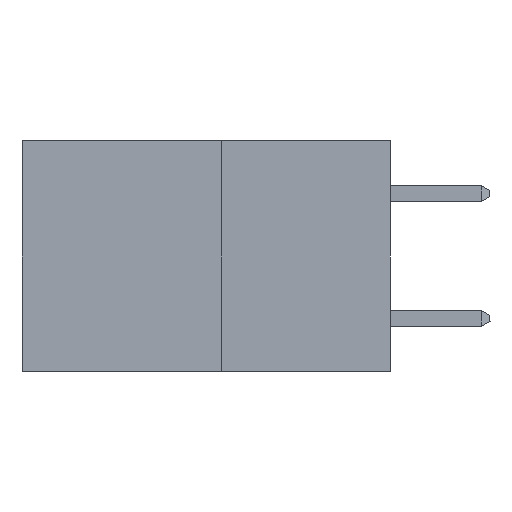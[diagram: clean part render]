
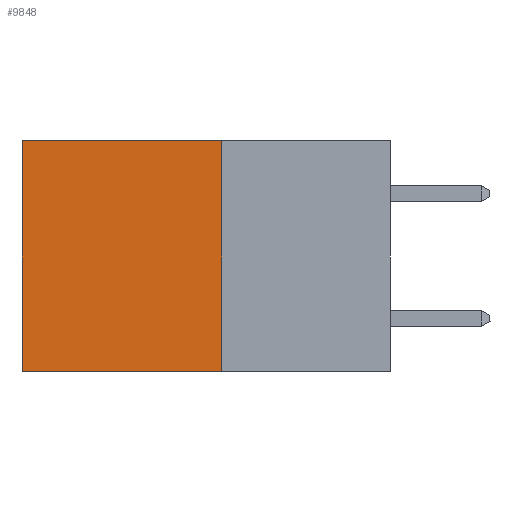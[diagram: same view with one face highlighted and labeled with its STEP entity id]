
A CAD part, left-side view. The second image highlights one B-rep face of the part: STEP entity #9848.
In plain terms, the highlighted planar face has unit normal (-1, 0, 0).
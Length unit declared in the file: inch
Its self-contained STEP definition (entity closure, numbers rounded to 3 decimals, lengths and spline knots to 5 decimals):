
#605 = ORIENTED_EDGE ( 'NONE', *, *, #17649, .T. ) ;
#949 = DIRECTION ( 'NONE',  ( 0., 1., 0. ) ) ;
#3124 = LINE ( 'NONE', #20658, #3784 ) ;
#3193 = FACE_OUTER_BOUND ( 'NONE', #20504, .T. ) ;
#3784 = VECTOR ( 'NONE', #10725, 39.37008 ) ;
#6838 = VERTEX_POINT ( 'NONE', #23692 ) ;
#7092 = AXIS2_PLACEMENT_3D ( 'NONE', #11351, #11276, #11159 ) ;
#8604 = VERTEX_POINT ( 'NONE', #24781 ) ;
#8710 = CARTESIAN_POINT ( 'NONE',  ( 0.277, 0.27, -0.37 ) ) ;
#9660 = VERTEX_POINT ( 'NONE', #15982 ) ;
#9848 = ADVANCED_FACE ( 'NONE', ( #3193 ), #11523, .F. ) ;
#10445 = DIRECTION ( 'NONE',  ( 0., 0., -1. ) ) ;
#10725 = DIRECTION ( 'NONE',  ( 0., 0., -1. ) ) ;
#11159 = DIRECTION ( 'NONE',  ( 0., 0., -1. ) ) ;
#11276 = DIRECTION ( 'NONE',  ( 1., 0., 0. ) ) ;
#11351 = CARTESIAN_POINT ( 'NONE',  ( 0.277, 0.27, -0.37 ) ) ;
#11523 = PLANE ( 'NONE',  #7092 ) ;
#11904 = LINE ( 'NONE', #23407, #21879 ) ;
#12302 = VECTOR ( 'NONE', #24926, 39.37008 ) ;
#13398 = ORIENTED_EDGE ( 'NONE', *, *, #17826, .T. ) ;
#13601 = EDGE_CURVE ( 'NONE', #23421, #9660, #3124, .T. ) ;
#14498 = CARTESIAN_POINT ( 'NONE',  ( 0.277, 0.59, -0.37 ) ) ;
#15982 = CARTESIAN_POINT ( 'NONE',  ( 0.277, 0.27, -0.37 ) ) ;
#16890 = LINE ( 'NONE', #14498, #20915 ) ;
#17649 = EDGE_CURVE ( 'NONE', #8604, #6838, #16890, .T. ) ;
#17826 = EDGE_CURVE ( 'NONE', #23421, #8604, #11904, .T. ) ;
#18219 = LINE ( 'NONE', #8710, #12302 ) ;
#19311 = ORIENTED_EDGE ( 'NONE', *, *, #25629, .F. ) ;
#20504 = EDGE_LOOP ( 'NONE', ( #605, #19311, #24139, #13398 ) ) ;
#20658 = CARTESIAN_POINT ( 'NONE',  ( 0.277, 0.27, -0.37 ) ) ;
#20915 = VECTOR ( 'NONE', #10445, 39.37008 ) ;
#21879 = VECTOR ( 'NONE', #949, 39.37008 ) ;
#23407 = CARTESIAN_POINT ( 'NONE',  ( 0.277, 0.27, 0. ) ) ;
#23421 = VERTEX_POINT ( 'NONE', #24371 ) ;
#23692 = CARTESIAN_POINT ( 'NONE',  ( 0.277, 0.59, -0.37 ) ) ;
#24139 = ORIENTED_EDGE ( 'NONE', *, *, #13601, .F. ) ;
#24371 = CARTESIAN_POINT ( 'NONE',  ( 0.277, 0.27, 0. ) ) ;
#24781 = CARTESIAN_POINT ( 'NONE',  ( 0.277, 0.59, 0. ) ) ;
#24926 = DIRECTION ( 'NONE',  ( 0., 1., 0. ) ) ;
#25629 = EDGE_CURVE ( 'NONE', #9660, #6838, #18219, .T. ) ;
